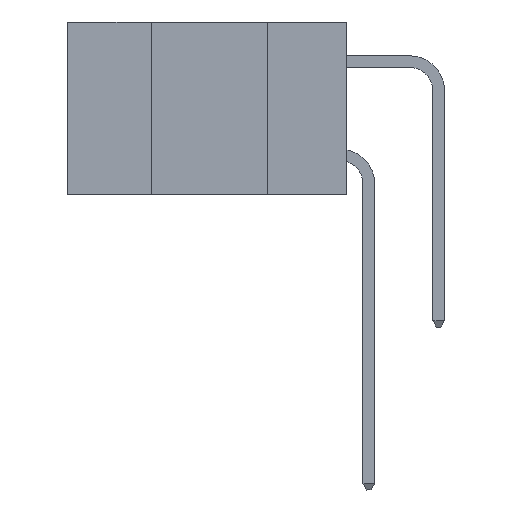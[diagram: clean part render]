
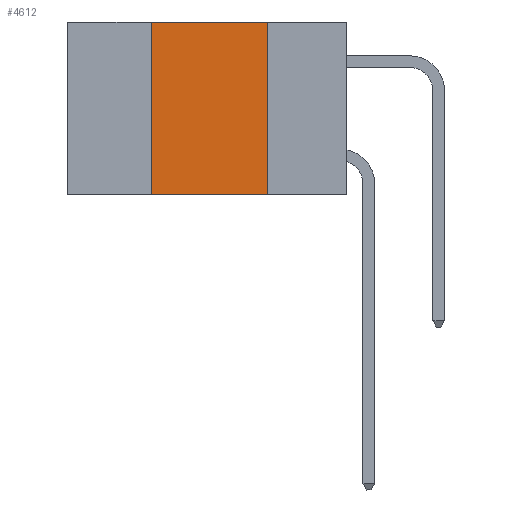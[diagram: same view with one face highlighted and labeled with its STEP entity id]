
A CAD part, left-side view. The second image highlights one B-rep face of the part: STEP entity #4612.
In plain terms, the highlighted planar face has unit normal (-1, 0, 0).
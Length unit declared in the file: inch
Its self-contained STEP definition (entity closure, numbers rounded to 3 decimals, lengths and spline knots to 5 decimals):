
#1046 = EDGE_CURVE ( 'NONE', #3159, #8768, #6102, .T. ) ;
#1476 = CARTESIAN_POINT ( 'NONE',  ( 0., 0.42, -0.37 ) ) ;
#2488 = CARTESIAN_POINT ( 'NONE',  ( 0., 0.42, 0. ) ) ;
#2789 = EDGE_CURVE ( 'NONE', #3159, #7205, #8371, .T. ) ;
#3159 = VERTEX_POINT ( 'NONE', #1476 ) ;
#4299 = CARTESIAN_POINT ( 'NONE',  ( 0., 0.6, -0.37 ) ) ;
#4612 = ADVANCED_FACE ( 'NONE', ( #21600 ), #24169, .F. ) ;
#6102 = LINE ( 'NONE', #2488, #20487 ) ;
#6138 = DIRECTION ( 'NONE',  ( 0., -1., 0. ) ) ;
#7205 = VERTEX_POINT ( 'NONE', #20643 ) ;
#7392 = ORIENTED_EDGE ( 'NONE', *, *, #2789, .T. ) ;
#8371 = LINE ( 'NONE', #4299, #17684 ) ;
#8768 = VERTEX_POINT ( 'NONE', #20722 ) ;
#9240 = DIRECTION ( 'NONE',  ( 1., 0., 0. ) ) ;
#9555 = ORIENTED_EDGE ( 'NONE', *, *, #13205, .F. ) ;
#9556 = VECTOR ( 'NONE', #15704, 39.37008 ) ;
#12190 = EDGE_CURVE ( 'NONE', #20696, #7205, #13580, .T. ) ;
#13053 = EDGE_LOOP ( 'NONE', ( #21063, #9555, #23631, #7392 ) ) ;
#13205 = EDGE_CURVE ( 'NONE', #8768, #20696, #14403, .T. ) ;
#13580 = LINE ( 'NONE', #20437, #18092 ) ;
#14403 = LINE ( 'NONE', #15627, #9556 ) ;
#15627 = CARTESIAN_POINT ( 'NONE',  ( 0., 0.6, 0. ) ) ;
#15704 = DIRECTION ( 'NONE',  ( 0., -1., 0. ) ) ;
#17234 = CARTESIAN_POINT ( 'NONE',  ( 0., 0.17, 0. ) ) ;
#17684 = VECTOR ( 'NONE', #6138, 39.37008 ) ;
#18092 = VECTOR ( 'NONE', #22318, 39.37008 ) ;
#20437 = CARTESIAN_POINT ( 'NONE',  ( 0., 0.17, 0. ) ) ;
#20487 = VECTOR ( 'NONE', #21162, 39.37008 ) ;
#20511 = CARTESIAN_POINT ( 'NONE',  ( 0., 0.6, 0. ) ) ;
#20643 = CARTESIAN_POINT ( 'NONE',  ( 0., 0.17, -0.37 ) ) ;
#20696 = VERTEX_POINT ( 'NONE', #17234 ) ;
#20722 = CARTESIAN_POINT ( 'NONE',  ( 0., 0.42, 0. ) ) ;
#21063 = ORIENTED_EDGE ( 'NONE', *, *, #12190, .F. ) ;
#21162 = DIRECTION ( 'NONE',  ( 0., 0., 1. ) ) ;
#21600 = FACE_OUTER_BOUND ( 'NONE', #13053, .T. ) ;
#22318 = DIRECTION ( 'NONE',  ( 0., 0., -1. ) ) ;
#22385 = DIRECTION ( 'NONE',  ( 0., 0., -1. ) ) ;
#23554 = AXIS2_PLACEMENT_3D ( 'NONE', #20511, #9240, #22385 ) ;
#23631 = ORIENTED_EDGE ( 'NONE', *, *, #1046, .F. ) ;
#24169 = PLANE ( 'NONE',  #23554 ) ;
